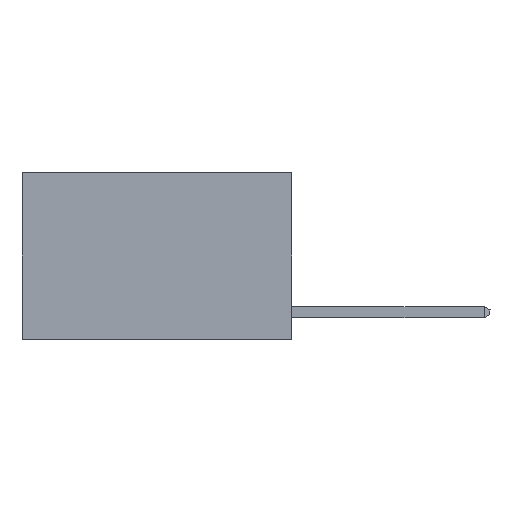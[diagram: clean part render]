
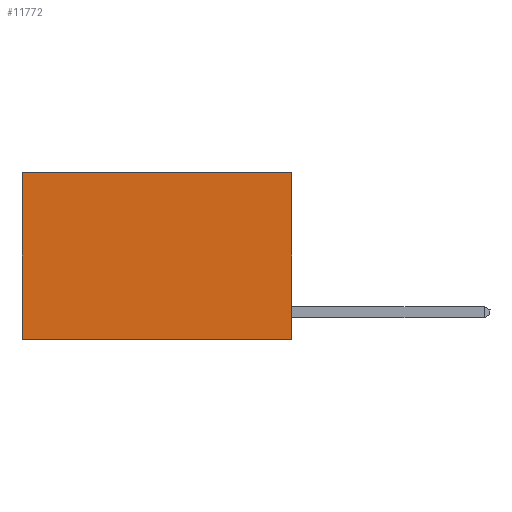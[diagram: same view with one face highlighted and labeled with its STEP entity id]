
A CAD part, left-side view. The second image highlights one B-rep face of the part: STEP entity #11772.
In plain terms, the highlighted planar face has unit normal (-1, 0, 0).
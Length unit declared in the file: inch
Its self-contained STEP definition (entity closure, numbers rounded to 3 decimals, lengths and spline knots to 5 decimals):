
#221 = CARTESIAN_POINT ( 'NONE',  ( 0.2625, 0., -0.37 ) ) ;
#422 = CARTESIAN_POINT ( 'NONE',  ( 0.2625, 0., 0. ) ) ;
#473 = FACE_OUTER_BOUND ( 'NONE', #5592, .T. ) ;
#853 = LINE ( 'NONE', #10322, #8952 ) ;
#1525 = DIRECTION ( 'NONE',  ( 0., 0., -1. ) ) ;
#2090 = EDGE_CURVE ( 'NONE', #5319, #5835, #9213, .T. ) ;
#2473 = ORIENTED_EDGE ( 'NONE', *, *, #9249, .T. ) ;
#2487 = ORIENTED_EDGE ( 'NONE', *, *, #9019, .F. ) ;
#2633 = ORIENTED_EDGE ( 'NONE', *, *, #2090, .F. ) ;
#2739 = ORIENTED_EDGE ( 'NONE', *, *, #6850, .T. ) ;
#2864 = AXIS2_PLACEMENT_3D ( 'NONE', #11400, #5115, #12462 ) ;
#2896 = VERTEX_POINT ( 'NONE', #7900 ) ;
#2977 = PLANE ( 'NONE',  #2864 ) ;
#4634 = CARTESIAN_POINT ( 'NONE',  ( 0.2625, 0., -0.37 ) ) ;
#4643 = LINE ( 'NONE', #6280, #12366 ) ;
#5115 = DIRECTION ( 'NONE',  ( 1., 0., 0. ) ) ;
#5319 = VERTEX_POINT ( 'NONE', #422 ) ;
#5592 = EDGE_LOOP ( 'NONE', ( #2473, #2487, #2633, #2739 ) ) ;
#5835 = VERTEX_POINT ( 'NONE', #221 ) ;
#6280 = CARTESIAN_POINT ( 'NONE',  ( 0.2625, 0., 0. ) ) ;
#6850 = EDGE_CURVE ( 'NONE', #5319, #12844, #4643, .T. ) ;
#7900 = CARTESIAN_POINT ( 'NONE',  ( 0.2625, 0.6, -0.37 ) ) ;
#8093 = CARTESIAN_POINT ( 'NONE',  ( 0.2625, 0., 0. ) ) ;
#8952 = VECTOR ( 'NONE', #11367, 39.37008 ) ;
#9019 = EDGE_CURVE ( 'NONE', #5835, #2896, #9774, .T. ) ;
#9213 = LINE ( 'NONE', #8093, #11657 ) ;
#9249 = EDGE_CURVE ( 'NONE', #12844, #2896, #853, .T. ) ;
#9774 = LINE ( 'NONE', #4634, #11891 ) ;
#10322 = CARTESIAN_POINT ( 'NONE',  ( 0.2625, 0.6, 0. ) ) ;
#10642 = CARTESIAN_POINT ( 'NONE',  ( 0.2625, 0.6, 0. ) ) ;
#11367 = DIRECTION ( 'NONE',  ( 0., 0., -1. ) ) ;
#11400 = CARTESIAN_POINT ( 'NONE',  ( 0.2625, 0., 0. ) ) ;
#11657 = VECTOR ( 'NONE', #1525, 39.37008 ) ;
#11772 = ADVANCED_FACE ( 'NONE', ( #473 ), #2977, .F. ) ;
#11891 = VECTOR ( 'NONE', #13118, 39.37008 ) ;
#12366 = VECTOR ( 'NONE', #12590, 39.37008 ) ;
#12462 = DIRECTION ( 'NONE',  ( 0., 0., -1. ) ) ;
#12590 = DIRECTION ( 'NONE',  ( 0., 1., 0. ) ) ;
#12844 = VERTEX_POINT ( 'NONE', #10642 ) ;
#13118 = DIRECTION ( 'NONE',  ( 0., 1., 0. ) ) ;
